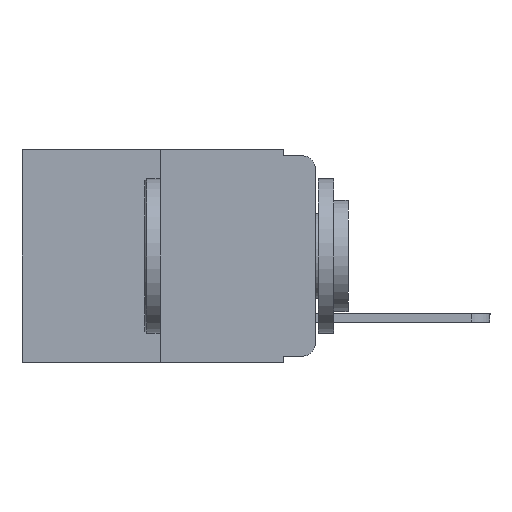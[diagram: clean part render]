
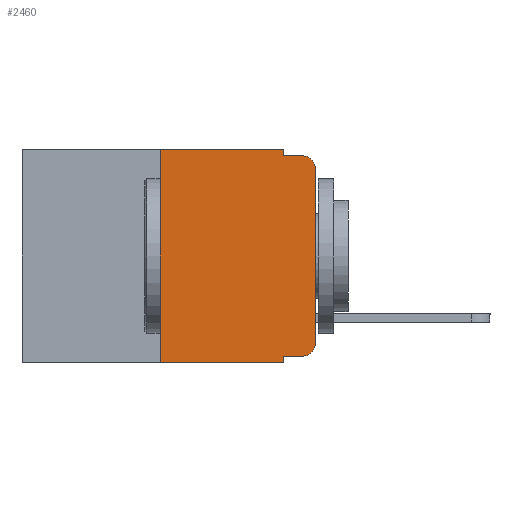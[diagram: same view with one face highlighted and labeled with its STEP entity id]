
A CAD part, left-side view. The second image highlights one B-rep face of the part: STEP entity #2460.
In plain terms, the highlighted planar face has unit normal (-1, 0, 0).
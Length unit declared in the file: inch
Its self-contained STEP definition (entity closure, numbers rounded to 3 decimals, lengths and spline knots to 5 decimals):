
#182 = AXIS2_PLACEMENT_3D ( 'NONE', #17825, #8765, #19312 ) ;
#252 = ORIENTED_EDGE ( 'NONE', *, *, #7564, .F. ) ;
#500 = AXIS2_PLACEMENT_3D ( 'NONE', #7344, #18094, #9051 ) ;
#567 = ORIENTED_EDGE ( 'NONE', *, *, #5930, .T. ) ;
#944 = CIRCLE ( 'NONE', #500, 0.02 ) ;
#1346 = DIRECTION ( 'NONE',  ( 0., 0., -1. ) ) ;
#1414 = VERTEX_POINT ( 'NONE', #18219 ) ;
#1491 = VECTOR ( 'NONE', #12467, 39.37008 ) ;
#1667 = CARTESIAN_POINT ( 'NONE',  ( 0., 0.25, -0.343 ) ) ;
#1963 = ORIENTED_EDGE ( 'NONE', *, *, #17247, .T. ) ;
#2148 = VERTEX_POINT ( 'NONE', #2730 ) ;
#2460 = ADVANCED_FACE ( 'NONE', ( #13466 ), #17091, .F. ) ;
#2638 = CARTESIAN_POINT ( 'NONE',  ( 0., 0., -0.313 ) ) ;
#2730 = CARTESIAN_POINT ( 'NONE',  ( 0., 0.051, 0. ) ) ;
#3341 = DIRECTION ( 'NONE',  ( 1., 0., 0. ) ) ;
#3916 = EDGE_CURVE ( 'NONE', #6357, #2148, #18691, .T. ) ;
#4012 = VECTOR ( 'NONE', #12864, 39.37008 ) ;
#4313 = VERTEX_POINT ( 'NONE', #2638 ) ;
#4939 = VERTEX_POINT ( 'NONE', #7653 ) ;
#5237 = VECTOR ( 'NONE', #8918, 39.37008 ) ;
#5361 = ORIENTED_EDGE ( 'NONE', *, *, #17613, .F. ) ;
#5930 = EDGE_CURVE ( 'NONE', #14215, #18312, #17210, .T. ) ;
#6185 = VERTEX_POINT ( 'NONE', #18804 ) ;
#6357 = VERTEX_POINT ( 'NONE', #16460 ) ;
#6782 = EDGE_CURVE ( 'NONE', #14215, #6357, #7800, .T. ) ;
#6889 = VECTOR ( 'NONE', #11519, 39.37008 ) ;
#6901 = ORIENTED_EDGE ( 'NONE', *, *, #18431, .T. ) ;
#7115 = VECTOR ( 'NONE', #11771, 39.37008 ) ;
#7344 = CARTESIAN_POINT ( 'NONE',  ( 0., 0.02, -0.03 ) ) ;
#7407 = EDGE_LOOP ( 'NONE', ( #6901, #14746, #252, #17051, #18245, #10595, #567, #5361, #1963, #16839 ) ) ;
#7564 = EDGE_CURVE ( 'NONE', #4939, #16796, #9070, .T. ) ;
#7653 = CARTESIAN_POINT ( 'NONE',  ( 0., 0.051, -0.01 ) ) ;
#7800 = LINE ( 'NONE', #11812, #19020 ) ;
#8765 = DIRECTION ( 'NONE',  ( -1., 0., 0. ) ) ;
#8918 = DIRECTION ( 'NONE',  ( 0., -1., 0. ) ) ;
#9034 = CARTESIAN_POINT ( 'NONE',  ( 0., 0.051, -0.343 ) ) ;
#9051 = DIRECTION ( 'NONE',  ( 0., 0., -1. ) ) ;
#9070 = LINE ( 'NONE', #20149, #4012 ) ;
#9689 = EDGE_CURVE ( 'NONE', #2148, #4939, #15393, .T. ) ;
#10595 = ORIENTED_EDGE ( 'NONE', *, *, #6782, .F. ) ;
#10653 = LINE ( 'NONE', #10910, #1491 ) ;
#10910 = CARTESIAN_POINT ( 'NONE',  ( 0., 0., 0. ) ) ;
#11326 = CARTESIAN_POINT ( 'NONE',  ( 0., 0.051, -0.333 ) ) ;
#11519 = DIRECTION ( 'NONE',  ( 0., -1., 0. ) ) ;
#11628 = CARTESIAN_POINT ( 'NONE',  ( 0., 0.473, 0. ) ) ;
#11771 = DIRECTION ( 'NONE',  ( 0., 0., -1. ) ) ;
#11788 = AXIS2_PLACEMENT_3D ( 'NONE', #18754, #3341, #14628 ) ;
#11812 = CARTESIAN_POINT ( 'NONE',  ( 0., 0.25, 0. ) ) ;
#12467 = DIRECTION ( 'NONE',  ( 0., 0., 1. ) ) ;
#12846 = LINE ( 'NONE', #20362, #20169 ) ;
#12864 = DIRECTION ( 'NONE',  ( 0., -1., 0. ) ) ;
#13466 = FACE_OUTER_BOUND ( 'NONE', #7407, .T. ) ;
#13952 = CIRCLE ( 'NONE', #182, 0.02 ) ;
#13968 = VECTOR ( 'NONE', #18285, 39.37008 ) ;
#14215 = VERTEX_POINT ( 'NONE', #1667 ) ;
#14628 = DIRECTION ( 'NONE',  ( 0., 0., -1. ) ) ;
#14746 = ORIENTED_EDGE ( 'NONE', *, *, #20052, .T. ) ;
#14889 = LINE ( 'NONE', #16805, #13968 ) ;
#15010 = VERTEX_POINT ( 'NONE', #11326 ) ;
#15393 = LINE ( 'NONE', #20590, #7115 ) ;
#16460 = CARTESIAN_POINT ( 'NONE',  ( 0., 0.25, 0. ) ) ;
#16796 = VERTEX_POINT ( 'NONE', #20389 ) ;
#16805 = CARTESIAN_POINT ( 'NONE',  ( 0., 0.051, -0.333 ) ) ;
#16839 = ORIENTED_EDGE ( 'NONE', *, *, #17837, .T. ) ;
#17051 = ORIENTED_EDGE ( 'NONE', *, *, #9689, .F. ) ;
#17091 = PLANE ( 'NONE',  #11788 ) ;
#17210 = LINE ( 'NONE', #19456, #5237 ) ;
#17247 = EDGE_CURVE ( 'NONE', #15010, #1414, #14889, .T. ) ;
#17613 = EDGE_CURVE ( 'NONE', #15010, #18312, #12846, .T. ) ;
#17825 = CARTESIAN_POINT ( 'NONE',  ( 0., 0.02, -0.313 ) ) ;
#17837 = EDGE_CURVE ( 'NONE', #1414, #4313, #13952, .T. ) ;
#18094 = DIRECTION ( 'NONE',  ( -1., 0., 0. ) ) ;
#18219 = CARTESIAN_POINT ( 'NONE',  ( 0., 0.02, -0.333 ) ) ;
#18245 = ORIENTED_EDGE ( 'NONE', *, *, #3916, .F. ) ;
#18285 = DIRECTION ( 'NONE',  ( 0., -1., 0. ) ) ;
#18312 = VERTEX_POINT ( 'NONE', #9034 ) ;
#18431 = EDGE_CURVE ( 'NONE', #4313, #6185, #10653, .T. ) ;
#18691 = LINE ( 'NONE', #11628, #6889 ) ;
#18754 = CARTESIAN_POINT ( 'NONE',  ( 0., 0.473, 0. ) ) ;
#18804 = CARTESIAN_POINT ( 'NONE',  ( 0., 0., -0.03 ) ) ;
#19020 = VECTOR ( 'NONE', #20638, 39.37008 ) ;
#19312 = DIRECTION ( 'NONE',  ( 0., 0., -1. ) ) ;
#19456 = CARTESIAN_POINT ( 'NONE',  ( 0., 0.473, -0.343 ) ) ;
#20052 = EDGE_CURVE ( 'NONE', #6185, #16796, #944, .T. ) ;
#20149 = CARTESIAN_POINT ( 'NONE',  ( 0., 0.051, -0.01 ) ) ;
#20169 = VECTOR ( 'NONE', #1346, 39.37008 ) ;
#20362 = CARTESIAN_POINT ( 'NONE',  ( 0., 0.051, 0. ) ) ;
#20389 = CARTESIAN_POINT ( 'NONE',  ( 0., 0.02, -0.01 ) ) ;
#20590 = CARTESIAN_POINT ( 'NONE',  ( 0., 0.051, 0. ) ) ;
#20638 = DIRECTION ( 'NONE',  ( 0., 0., 1. ) ) ;
